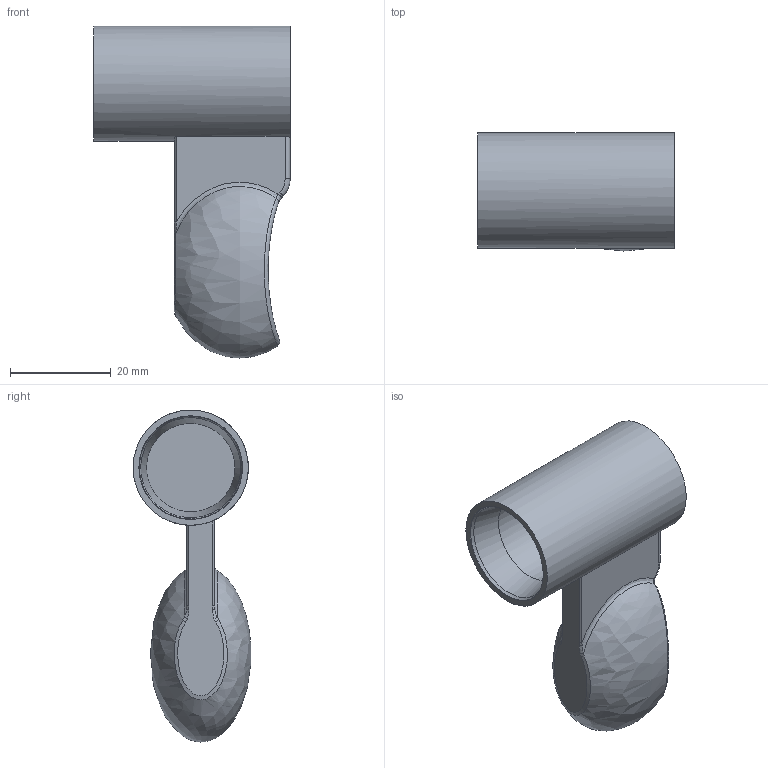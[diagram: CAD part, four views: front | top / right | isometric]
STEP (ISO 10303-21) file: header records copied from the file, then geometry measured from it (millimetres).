
FILE_DESCRIPTION(('FreeCAD Model'),'2;1');
FILE_NAME('charging handle long.step','2020-04-26T15:41:00',('Author'),(''), 'Open CASCADE STEP processor 6.8','FreeCAD','Unknown');
FILE_SCHEMA(('AUTOMOTIVE_DESIGN_CC2 { 1 2 10303 214 -1 1 5 4 }'));
Length unit declared in the file: millimetre
Products named in the file (1): Chamfer002
Bounding box: 39 x 23.4 x 65.95 mm (x, y, z)
Volume: 19579.2 mm3; surface area: 7551.5 mm2
Topology: 1 solids, 1 shells, 40 faces, 98 edges, 60 vertices
Faces by surface type: bspline 21, plane 11, cylinder 5, cone 2, torus 1
Full cylindrical faces by diameter (mm): 17.6 x1, 22.9 x1
Entity records: 5900 total; most frequent: CARTESIAN_POINT 4319, ORIENTED_EDGE 192, PCURVE 192, DEFINITIONAL_REPRESENTATION 192, B_SPLINE_CURVE_WITH_KNOTS 173, DIRECTION 167, EDGE_CURVE 96, SURFACE_CURVE 90
